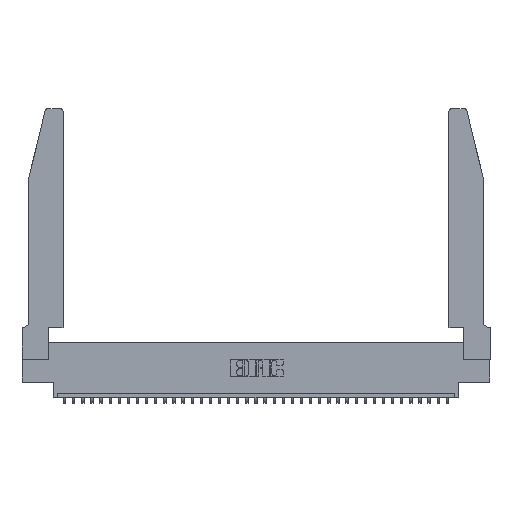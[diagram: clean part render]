
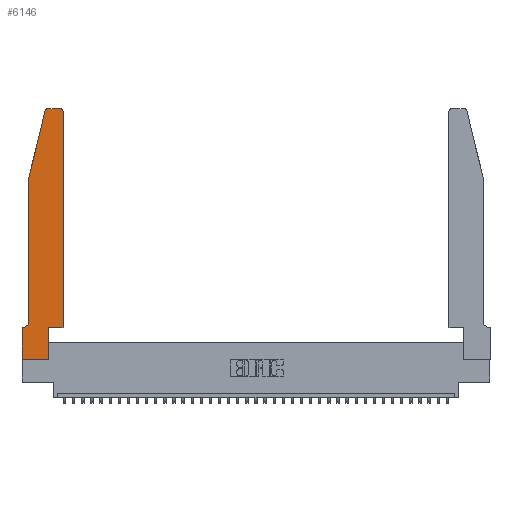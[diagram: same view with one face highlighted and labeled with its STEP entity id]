
A CAD part, top view. The second image highlights one B-rep face of the part: STEP entity #6146.
In plain terms, the highlighted planar face has unit normal (0, 0, 1).
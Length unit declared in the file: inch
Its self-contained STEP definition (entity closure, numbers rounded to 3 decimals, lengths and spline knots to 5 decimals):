
#562 = DIRECTION ( 'NONE',  ( -1., 0., 0. ) ) ;
#961 = CARTESIAN_POINT ( 'NONE',  ( 0.284, 2.75, 0.37 ) ) ;
#1042 = LINE ( 'NONE', #25119, #30243 ) ;
#2638 = CARTESIAN_POINT ( 'NONE',  ( 0., 0.35, 0.37 ) ) ;
#2698 = DIRECTION ( 'NONE',  ( 1., 0., 0. ) ) ;
#2932 = DIRECTION ( 'NONE',  ( 0., -1., 0. ) ) ;
#3051 = CARTESIAN_POINT ( 'NONE',  ( 0., 0., 0.37 ) ) ;
#3324 = LINE ( 'NONE', #23054, #25824 ) ;
#3522 = CARTESIAN_POINT ( 'NONE',  ( 0.2865, 0., 0.37 ) ) ;
#3613 = VECTOR ( 'NONE', #6975, 39.37008 ) ;
#3784 = VECTOR ( 'NONE', #8277, 39.37008 ) ;
#4007 = ORIENTED_EDGE ( 'NONE', *, *, #11670, .T. ) ;
#4379 = CARTESIAN_POINT ( 'NONE',  ( 0.0055, 0.35, 0.37 ) ) ;
#4817 = LINE ( 'NONE', #3051, #21388 ) ;
#4992 = CARTESIAN_POINT ( 'NONE',  ( 0.284, 2.72, 0.37 ) ) ;
#5123 = CARTESIAN_POINT ( 'NONE',  ( 0.4505, 0.35, 0.37 ) ) ;
#6143 = EDGE_CURVE ( 'NONE', #8744, #15807, #28767, .T. ) ;
#6146 = ADVANCED_FACE ( 'NONE', ( #20177 ), #8179, .T. ) ;
#6205 = DIRECTION ( 'NONE',  ( 0., 0., -1. ) ) ;
#6381 = ORIENTED_EDGE ( 'NONE', *, *, #20084, .T. ) ;
#6920 = CARTESIAN_POINT ( 'NONE',  ( 0.4505, 2.72, 0.37 ) ) ;
#6975 = DIRECTION ( 'NONE',  ( -1., 0., 0. ) ) ;
#7009 = VERTEX_POINT ( 'NONE', #9986 ) ;
#7460 = CARTESIAN_POINT ( 'NONE',  ( 0.2865, 0.35, 0.37 ) ) ;
#7822 = DIRECTION ( 'NONE',  ( 1., 0., 0. ) ) ;
#7966 = DIRECTION ( 'NONE',  ( -1., 0., 0. ) ) ;
#8109 = AXIS2_PLACEMENT_3D ( 'NONE', #2638, #22688, #7822 ) ;
#8179 = PLANE ( 'NONE',  #8109 ) ;
#8226 = VECTOR ( 'NONE', #35660, 39.37008 ) ;
#8277 = DIRECTION ( 'NONE',  ( 0., 1., 0. ) ) ;
#8573 = LINE ( 'NONE', #11874, #3613 ) ;
#8744 = VERTEX_POINT ( 'NONE', #3522 ) ;
#9655 = LINE ( 'NONE', #5123, #3784 ) ;
#9986 = CARTESIAN_POINT ( 'NONE',  ( 0.0755, 2., 0.37 ) ) ;
#10184 = VERTEX_POINT ( 'NONE', #23887 ) ;
#10222 = ORIENTED_EDGE ( 'NONE', *, *, #21297, .T. ) ;
#10245 = EDGE_CURVE ( 'NONE', #36528, #31128, #1042, .T. ) ;
#11193 = ORIENTED_EDGE ( 'NONE', *, *, #34905, .T. ) ;
#11325 = CARTESIAN_POINT ( 'NONE',  ( 0.25487, 2.72718, 0.37 ) ) ;
#11423 = EDGE_CURVE ( 'NONE', #15807, #10184, #17272, .T. ) ;
#11670 = EDGE_CURVE ( 'NONE', #21666, #36528, #34780, .T. ) ;
#11874 = CARTESIAN_POINT ( 'NONE',  ( 0.0755, 0.35, 0.37 ) ) ;
#12061 = ORIENTED_EDGE ( 'NONE', *, *, #12476, .T. ) ;
#12338 = VECTOR ( 'NONE', #27138, 39.37008 ) ;
#12476 = EDGE_CURVE ( 'NONE', #14902, #8744, #18558, .T. ) ;
#12573 = VECTOR ( 'NONE', #16819, 39.37008 ) ;
#12871 = ORIENTED_EDGE ( 'NONE', *, *, #10245, .T. ) ;
#13006 = ORIENTED_EDGE ( 'NONE', *, *, #11423, .T. ) ;
#13102 = VERTEX_POINT ( 'NONE', #4379 ) ;
#14226 = DIRECTION ( 'NONE',  ( -0.239, -0.971, 0. ) ) ;
#14294 = EDGE_LOOP ( 'NONE', ( #12871, #27896, #10222, #16796, #26396, #6381, #33928, #12061, #33259, #13006, #11193, #4007 ) ) ;
#14309 = DIRECTION ( 'NONE',  ( 0., -1., 0. ) ) ;
#14531 = CARTESIAN_POINT ( 'NONE',  ( 0.0055, 0.42, 0.37 ) ) ;
#14902 = VERTEX_POINT ( 'NONE', #33413 ) ;
#14993 = CARTESIAN_POINT ( 'NONE',  ( 0.0755, 0.42, 0.37 ) ) ;
#15649 = LINE ( 'NONE', #22612, #26388 ) ;
#15807 = VERTEX_POINT ( 'NONE', #7460 ) ;
#16178 = AXIS2_PLACEMENT_3D ( 'NONE', #4992, #22637, #28200 ) ;
#16796 = ORIENTED_EDGE ( 'NONE', *, *, #34459, .T. ) ;
#16819 = DIRECTION ( 'NONE',  ( 0., 1., 0. ) ) ;
#17272 = LINE ( 'NONE', #32832, #12338 ) ;
#18558 = LINE ( 'NONE', #36535, #8226 ) ;
#20063 = AXIS2_PLACEMENT_3D ( 'NONE', #22513, #37131, #2698 ) ;
#20084 = EDGE_CURVE ( 'NONE', #13102, #24513, #8573, .T. ) ;
#20173 = CIRCLE ( 'NONE', #16178, 0.03 ) ;
#20177 = FACE_OUTER_BOUND ( 'NONE', #14294, .T. ) ;
#20663 = EDGE_CURVE ( 'NONE', #31128, #34496, #20173, .T. ) ;
#20831 = CARTESIAN_POINT ( 'NONE',  ( 0., 0.35, 0.37 ) ) ;
#21297 = EDGE_CURVE ( 'NONE', #34496, #7009, #15649, .T. ) ;
#21388 = VECTOR ( 'NONE', #2932, 39.37008 ) ;
#21666 = VERTEX_POINT ( 'NONE', #6920 ) ;
#22513 = CARTESIAN_POINT ( 'NONE',  ( 0.4205, 2.72, 0.37 ) ) ;
#22612 = CARTESIAN_POINT ( 'NONE',  ( 0.0755, 2., 0.37 ) ) ;
#22637 = DIRECTION ( 'NONE',  ( 0., 0., 1. ) ) ;
#22688 = DIRECTION ( 'NONE',  ( 0., 0., 1. ) ) ;
#23054 = CARTESIAN_POINT ( 'NONE',  ( 0.0755, 2., 0.37 ) ) ;
#23384 = AXIS2_PLACEMENT_3D ( 'NONE', #14531, #6205, #562 ) ;
#23414 = EDGE_CURVE ( 'NONE', #24513, #14902, #4817, .T. ) ;
#23887 = CARTESIAN_POINT ( 'NONE',  ( 0.4505, 0.35, 0.37 ) ) ;
#24126 = CIRCLE ( 'NONE', #23384, 0.07 ) ;
#24513 = VERTEX_POINT ( 'NONE', #20831 ) ;
#25119 = CARTESIAN_POINT ( 'NONE',  ( 0.2605, 2.75, 0.37 ) ) ;
#25824 = VECTOR ( 'NONE', #14309, 39.37008 ) ;
#26388 = VECTOR ( 'NONE', #14226, 39.37008 ) ;
#26396 = ORIENTED_EDGE ( 'NONE', *, *, #32647, .T. ) ;
#27138 = DIRECTION ( 'NONE',  ( 1., 0., 0. ) ) ;
#27896 = ORIENTED_EDGE ( 'NONE', *, *, #20663, .T. ) ;
#28200 = DIRECTION ( 'NONE',  ( 1., 0., 0. ) ) ;
#28767 = LINE ( 'NONE', #37069, #12573 ) ;
#30243 = VECTOR ( 'NONE', #7966, 39.37008 ) ;
#31128 = VERTEX_POINT ( 'NONE', #961 ) ;
#32647 = EDGE_CURVE ( 'NONE', #32743, #13102, #24126, .T. ) ;
#32743 = VERTEX_POINT ( 'NONE', #14993 ) ;
#32832 = CARTESIAN_POINT ( 'NONE',  ( 0.4505, 0.35, 0.37 ) ) ;
#33259 = ORIENTED_EDGE ( 'NONE', *, *, #6143, .T. ) ;
#33413 = CARTESIAN_POINT ( 'NONE',  ( 0., 0., 0.37 ) ) ;
#33928 = ORIENTED_EDGE ( 'NONE', *, *, #23414, .T. ) ;
#34459 = EDGE_CURVE ( 'NONE', #7009, #32743, #3324, .T. ) ;
#34496 = VERTEX_POINT ( 'NONE', #11325 ) ;
#34780 = CIRCLE ( 'NONE', #20063, 0.03 ) ;
#34905 = EDGE_CURVE ( 'NONE', #10184, #21666, #9655, .T. ) ;
#35411 = CARTESIAN_POINT ( 'NONE',  ( 0.4205, 2.75, 0.37 ) ) ;
#35660 = DIRECTION ( 'NONE',  ( 1., 0., 0. ) ) ;
#36528 = VERTEX_POINT ( 'NONE', #35411 ) ;
#36535 = CARTESIAN_POINT ( 'NONE',  ( 0., 0., 0.37 ) ) ;
#37069 = CARTESIAN_POINT ( 'NONE',  ( 0.2865, 0.35, 0.37 ) ) ;
#37131 = DIRECTION ( 'NONE',  ( 0., 0., 1. ) ) ;
